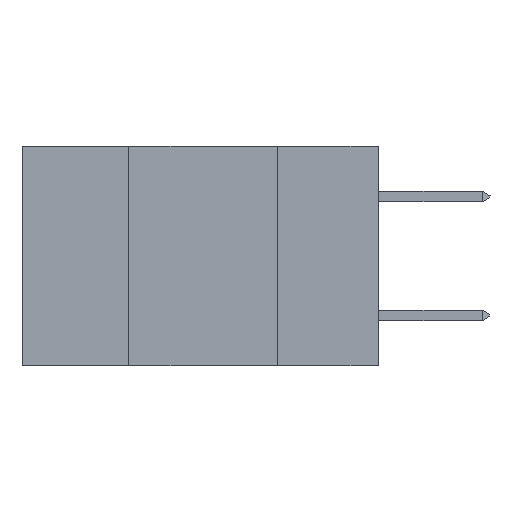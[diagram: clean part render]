
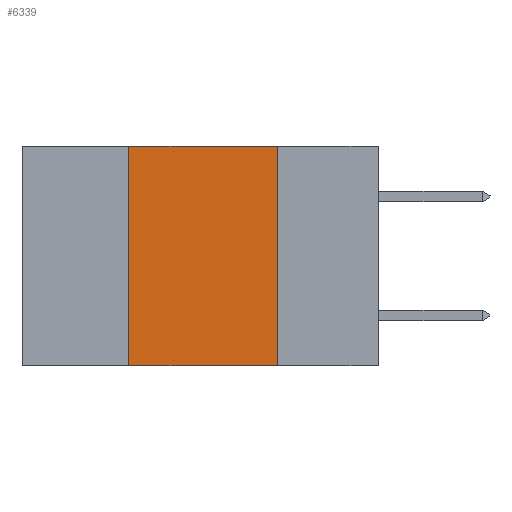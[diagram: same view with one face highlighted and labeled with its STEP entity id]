
A CAD part, left-side view. The second image highlights one B-rep face of the part: STEP entity #6339.
In plain terms, the highlighted planar face has unit normal (-1, 0, 0).
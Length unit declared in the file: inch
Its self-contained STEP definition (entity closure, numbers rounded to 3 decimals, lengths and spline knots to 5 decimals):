
#387 = EDGE_CURVE ( 'NONE', #7472, #467, #9379, .T. ) ;
#467 = VERTEX_POINT ( 'NONE', #6972 ) ;
#1119 = EDGE_CURVE ( 'NONE', #7524, #7472, #9010, .T. ) ;
#1766 = DIRECTION ( 'NONE',  ( 0., 0., -1. ) ) ;
#1960 = EDGE_CURVE ( 'NONE', #8998, #7524, #13042, .T. ) ;
#2435 = DIRECTION ( 'NONE',  ( 0., 0., 1. ) ) ;
#3286 = EDGE_CURVE ( 'NONE', #8998, #467, #17968, .T. ) ;
#4159 = PLANE ( 'NONE',  #6275 ) ;
#4295 = CARTESIAN_POINT ( 'NONE',  ( 0., 0.6, -0.37 ) ) ;
#4998 = ORIENTED_EDGE ( 'NONE', *, *, #1119, .F. ) ;
#5446 = FACE_OUTER_BOUND ( 'NONE', #13223, .T. ) ;
#6275 = AXIS2_PLACEMENT_3D ( 'NONE', #10056, #17716, #8767 ) ;
#6339 = ADVANCED_FACE ( 'NONE', ( #5446 ), #4159, .F. ) ;
#6972 = CARTESIAN_POINT ( 'NONE',  ( 0., 0.17, -0.37 ) ) ;
#7472 = VERTEX_POINT ( 'NONE', #15676 ) ;
#7524 = VERTEX_POINT ( 'NONE', #14254 ) ;
#7798 = CARTESIAN_POINT ( 'NONE',  ( 0., 0.6, 0. ) ) ;
#8767 = DIRECTION ( 'NONE',  ( 0., 0., -1. ) ) ;
#8998 = VERTEX_POINT ( 'NONE', #14183 ) ;
#9010 = LINE ( 'NONE', #7798, #14875 ) ;
#9017 = DIRECTION ( 'NONE',  ( 0., -1., 0. ) ) ;
#9379 = LINE ( 'NONE', #14067, #18466 ) ;
#10056 = CARTESIAN_POINT ( 'NONE',  ( 0., 0.6, 0. ) ) ;
#10701 = DIRECTION ( 'NONE',  ( 0., -1., 0. ) ) ;
#11582 = ORIENTED_EDGE ( 'NONE', *, *, #387, .F. ) ;
#11863 = ORIENTED_EDGE ( 'NONE', *, *, #3286, .T. ) ;
#13042 = LINE ( 'NONE', #14534, #15045 ) ;
#13223 = EDGE_LOOP ( 'NONE', ( #11582, #4998, #18007, #11863 ) ) ;
#14067 = CARTESIAN_POINT ( 'NONE',  ( 0., 0.17, -0.37 ) ) ;
#14183 = CARTESIAN_POINT ( 'NONE',  ( 0., 0.42, -0.37 ) ) ;
#14254 = CARTESIAN_POINT ( 'NONE',  ( 0., 0.42, 0. ) ) ;
#14534 = CARTESIAN_POINT ( 'NONE',  ( 0., 0.42, -0.37 ) ) ;
#14875 = VECTOR ( 'NONE', #10701, 39.37008 ) ;
#15045 = VECTOR ( 'NONE', #2435, 39.37008 ) ;
#15676 = CARTESIAN_POINT ( 'NONE',  ( 0., 0.17, 0. ) ) ;
#17716 = DIRECTION ( 'NONE',  ( 1., 0., 0. ) ) ;
#17968 = LINE ( 'NONE', #4295, #19642 ) ;
#18007 = ORIENTED_EDGE ( 'NONE', *, *, #1960, .F. ) ;
#18466 = VECTOR ( 'NONE', #1766, 39.37008 ) ;
#19642 = VECTOR ( 'NONE', #9017, 39.37008 ) ;
